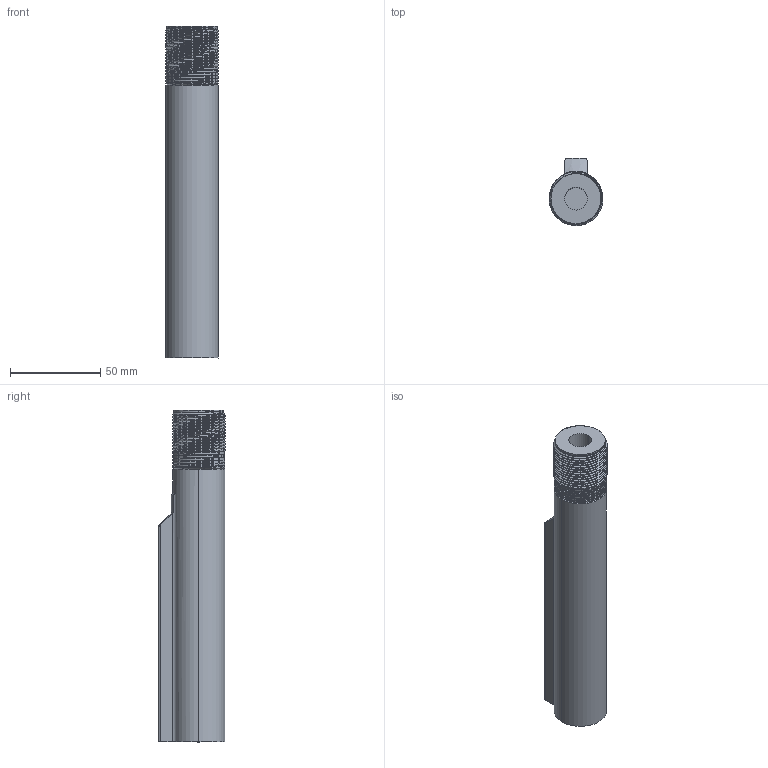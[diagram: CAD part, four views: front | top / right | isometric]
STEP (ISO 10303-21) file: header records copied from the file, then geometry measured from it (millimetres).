
FILE_DESCRIPTION (( 'STEP AP214' ), '1' );
FILE_NAME ('Dummy_Buffer_Tube.STEP', '2014-02-09T07:41:17', ( 'elpi' ), ( '' ), 'SwSTEP 2.0', 'SolidWorks 2013', '' );
FILE_SCHEMA (( 'AUTOMOTIVE_DESIGN' ));
Length unit declared in the file: inch
Products named in the file (1): Dummy_Buffer_Tube
Bounding box: 29.84 x 37.34 x 184.15 mm (x, y, z)
Volume: 108203.9 mm3; surface area: 30515.5 mm2
Topology: 1 solids, 1 shells, 228 faces, 643 edges, 422 vertices
Faces by surface type: cylinder 108, plane 60, bspline 46, cone 11, torus 3
Entity records: 23821 total; most frequent: CARTESIAN_POINT 18899, ORIENTED_EDGE 1286, DIRECTION 702, EDGE_CURVE 643, VERTEX_POINT 422, AXIS2_PLACEMENT_3D 261, B_SPLINE_CURVE_WITH_KNOTS 250, EDGE_LOOP 233
